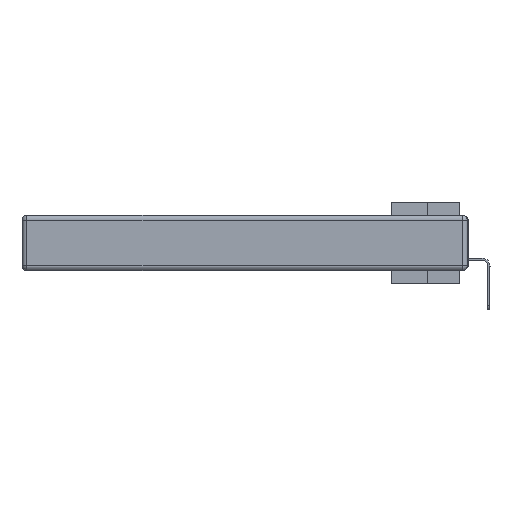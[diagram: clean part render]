
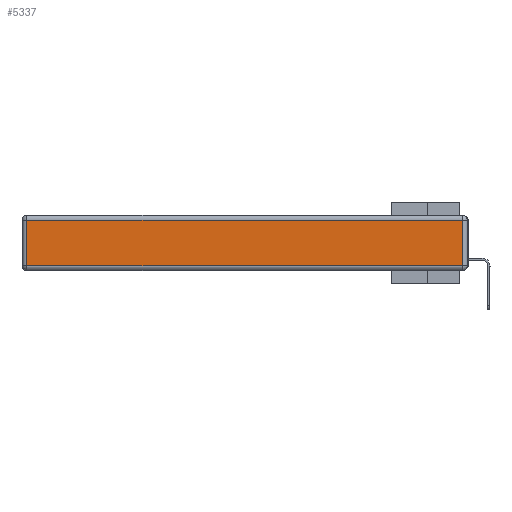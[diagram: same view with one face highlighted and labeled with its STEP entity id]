
A CAD part, left-side view. The second image highlights one B-rep face of the part: STEP entity #5337.
In plain terms, the highlighted planar face has unit normal (-1, 0, 0).
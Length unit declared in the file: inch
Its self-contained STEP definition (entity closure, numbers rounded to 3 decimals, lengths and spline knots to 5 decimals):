
#1768 = VERTEX_POINT ( 'NONE', #36591 ) ;
#2763 = DIRECTION ( 'NONE',  ( 0., 0., -1. ) ) ;
#5009 = DIRECTION ( 'NONE',  ( 0., -1., 0. ) ) ;
#5211 = CARTESIAN_POINT ( 'NONE',  ( 0., 2.72, -0.03 ) ) ;
#5295 = VERTEX_POINT ( 'NONE', #5211 ) ;
#5337 = ADVANCED_FACE ( 'NONE', ( #22247 ), #8854, .T. ) ;
#5909 = VERTEX_POINT ( 'NONE', #27126 ) ;
#6178 = CARTESIAN_POINT ( 'NONE',  ( 0., 2.72, -0.343 ) ) ;
#7482 = CARTESIAN_POINT ( 'NONE',  ( 0., 0., -0.313 ) ) ;
#8854 = PLANE ( 'NONE',  #17871 ) ;
#10443 = CARTESIAN_POINT ( 'NONE',  ( 0., 2.75, -0.03 ) ) ;
#11016 = EDGE_CURVE ( 'NONE', #5909, #1768, #20348, .T. ) ;
#11723 = ORIENTED_EDGE ( 'NONE', *, *, #30319, .T. ) ;
#12115 = LINE ( 'NONE', #10443, #21776 ) ;
#13135 = EDGE_CURVE ( 'NONE', #1768, #5295, #12115, .T. ) ;
#14686 = ORIENTED_EDGE ( 'NONE', *, *, #11016, .T. ) ;
#16350 = ORIENTED_EDGE ( 'NONE', *, *, #37695, .T. ) ;
#17800 = DIRECTION ( 'NONE',  ( 0., 0., 1. ) ) ;
#17871 = AXIS2_PLACEMENT_3D ( 'NONE', #33495, #18031, #39839 ) ;
#18031 = DIRECTION ( 'NONE',  ( -1., 0., 0. ) ) ;
#18217 = VECTOR ( 'NONE', #5009, 39.37008 ) ;
#18385 = EDGE_LOOP ( 'NONE', ( #16350, #14686, #31203, #11723 ) ) ;
#20348 = LINE ( 'NONE', #36295, #35921 ) ;
#21776 = VECTOR ( 'NONE', #35097, 39.37008 ) ;
#22247 = FACE_OUTER_BOUND ( 'NONE', #18385, .T. ) ;
#27126 = CARTESIAN_POINT ( 'NONE',  ( 0., 0.03, -0.313 ) ) ;
#28278 = LINE ( 'NONE', #6178, #35044 ) ;
#30185 = VERTEX_POINT ( 'NONE', #39333 ) ;
#30319 = EDGE_CURVE ( 'NONE', #5295, #30185, #28278, .T. ) ;
#31203 = ORIENTED_EDGE ( 'NONE', *, *, #13135, .T. ) ;
#33495 = CARTESIAN_POINT ( 'NONE',  ( 0., 0., -0.343 ) ) ;
#35044 = VECTOR ( 'NONE', #2763, 39.37008 ) ;
#35097 = DIRECTION ( 'NONE',  ( 0., 1., 0. ) ) ;
#35921 = VECTOR ( 'NONE', #17800, 39.37008 ) ;
#36295 = CARTESIAN_POINT ( 'NONE',  ( 0., 0.03, -0.343 ) ) ;
#36591 = CARTESIAN_POINT ( 'NONE',  ( 0., 0.03, -0.03 ) ) ;
#37695 = EDGE_CURVE ( 'NONE', #30185, #5909, #38180, .T. ) ;
#38180 = LINE ( 'NONE', #7482, #18217 ) ;
#39333 = CARTESIAN_POINT ( 'NONE',  ( 0., 2.72, -0.313 ) ) ;
#39839 = DIRECTION ( 'NONE',  ( 0., 0., 1. ) ) ;
